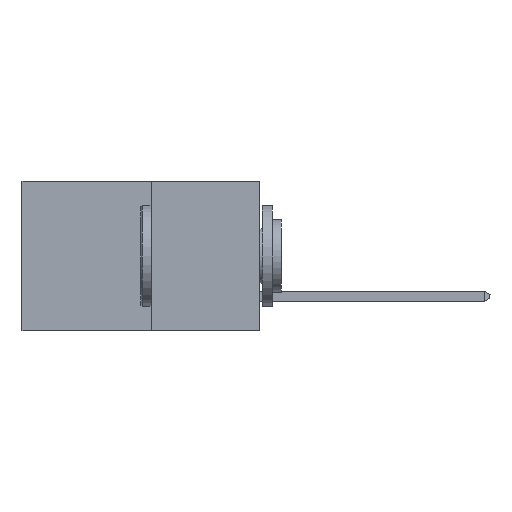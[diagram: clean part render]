
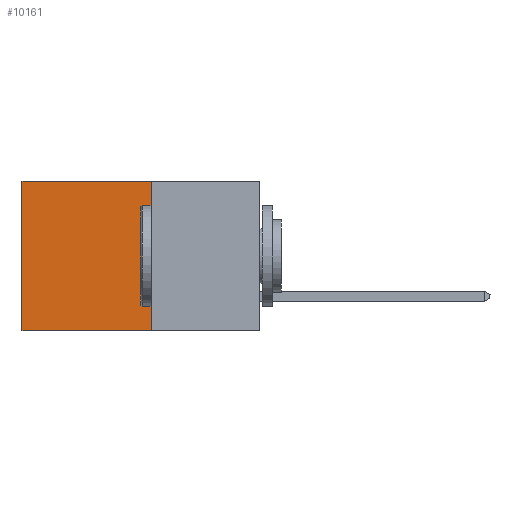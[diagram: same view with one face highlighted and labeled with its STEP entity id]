
A CAD part, left-side view. The second image highlights one B-rep face of the part: STEP entity #10161.
In plain terms, the highlighted planar face has unit normal (-1, 0, 0).
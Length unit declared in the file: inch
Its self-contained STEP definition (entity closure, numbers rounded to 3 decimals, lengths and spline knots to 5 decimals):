
#193 = CARTESIAN_POINT ( 'NONE',  ( 0.277, 0.27, -0.37 ) ) ;
#319 = VECTOR ( 'NONE', #2590, 39.37008 ) ;
#540 = DIRECTION ( 'NONE',  ( 0., 0., -1. ) ) ;
#559 = DIRECTION ( 'NONE',  ( 0., 1., 0. ) ) ;
#1105 = CARTESIAN_POINT ( 'NONE',  ( 0.277, 0.59, -0.37 ) ) ;
#1397 = VERTEX_POINT ( 'NONE', #12684 ) ;
#1408 = DIRECTION ( 'NONE',  ( 0., 1., 0. ) ) ;
#2096 = VECTOR ( 'NONE', #540, 39.37008 ) ;
#2590 = DIRECTION ( 'NONE',  ( 0., 0., -1. ) ) ;
#2982 = EDGE_LOOP ( 'NONE', ( #9208, #9670, #4411, #4657 ) ) ;
#3816 = VECTOR ( 'NONE', #1408, 39.37008 ) ;
#3997 = EDGE_CURVE ( 'NONE', #4721, #13552, #5151, .T. ) ;
#4258 = CARTESIAN_POINT ( 'NONE',  ( 0.277, 0.27, -0.37 ) ) ;
#4371 = VERTEX_POINT ( 'NONE', #6403 ) ;
#4411 = ORIENTED_EDGE ( 'NONE', *, *, #8007, .F. ) ;
#4657 = ORIENTED_EDGE ( 'NONE', *, *, #13892, .T. ) ;
#4721 = VERTEX_POINT ( 'NONE', #7715 ) ;
#5105 = CARTESIAN_POINT ( 'NONE',  ( 0.277, 0.27, 0. ) ) ;
#5151 = LINE ( 'NONE', #1105, #2096 ) ;
#5400 = DIRECTION ( 'NONE',  ( 0., 0., -1. ) ) ;
#6403 = CARTESIAN_POINT ( 'NONE',  ( 0.277, 0.27, -0.37 ) ) ;
#6924 = AXIS2_PLACEMENT_3D ( 'NONE', #4258, #12074, #5400 ) ;
#7715 = CARTESIAN_POINT ( 'NONE',  ( 0.277, 0.59, 0. ) ) ;
#8007 = EDGE_CURVE ( 'NONE', #1397, #4371, #12330, .T. ) ;
#8716 = PLANE ( 'NONE',  #6924 ) ;
#8808 = LINE ( 'NONE', #5105, #14338 ) ;
#9208 = ORIENTED_EDGE ( 'NONE', *, *, #3997, .T. ) ;
#9561 = CARTESIAN_POINT ( 'NONE',  ( 0.277, 0.59, -0.37 ) ) ;
#9670 = ORIENTED_EDGE ( 'NONE', *, *, #11243, .F. ) ;
#10161 = ADVANCED_FACE ( 'NONE', ( #12262 ), #8716, .F. ) ;
#11243 = EDGE_CURVE ( 'NONE', #4371, #13552, #13095, .T. ) ;
#12074 = DIRECTION ( 'NONE',  ( 1., 0., 0. ) ) ;
#12262 = FACE_OUTER_BOUND ( 'NONE', #2982, .T. ) ;
#12330 = LINE ( 'NONE', #12725, #319 ) ;
#12684 = CARTESIAN_POINT ( 'NONE',  ( 0.277, 0.27, 0. ) ) ;
#12725 = CARTESIAN_POINT ( 'NONE',  ( 0.277, 0.27, -0.37 ) ) ;
#13095 = LINE ( 'NONE', #193, #3816 ) ;
#13552 = VERTEX_POINT ( 'NONE', #9561 ) ;
#13892 = EDGE_CURVE ( 'NONE', #1397, #4721, #8808, .T. ) ;
#14338 = VECTOR ( 'NONE', #559, 39.37008 ) ;
